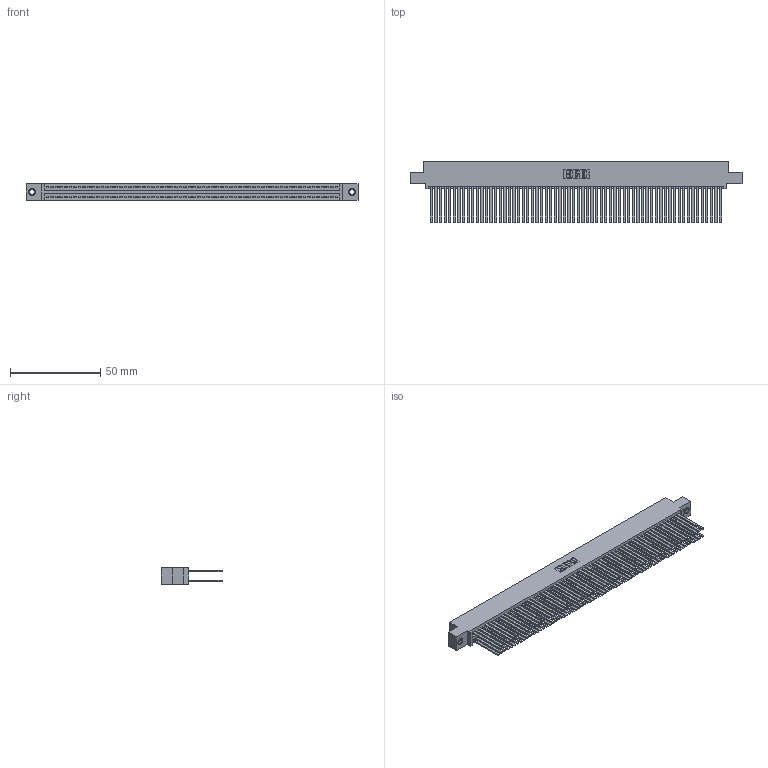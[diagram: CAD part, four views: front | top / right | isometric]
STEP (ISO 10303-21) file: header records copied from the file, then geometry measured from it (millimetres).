
FILE_DESCRIPTION (( 'STEP AP203' ), '1' );
FILE_NAME ('345-128-544-507.STEP', '2019-11-07T09:22:03', ( '' ), ( '' ), 'SwSTEP 2.0', 'SolidWorks 2016', '' );
FILE_SCHEMA (( 'CONFIG_CONTROL_DESIGN' ));
Length unit declared in the file: inch
Products named in the file (4): 345-128-544-507; 345-250-001_345-250-005-103; 345 Part_0.110 Offset - 0.156 Dia-TI; 345-292-001_345-293-144
Assembly tree (131 placements, depth 2):
  345-128-544-507
    345 Part_0.110 Offset - 0.156 Dia-TI
    345-292-001_345-293-144  x128
    345-250-001_345-250-005-103  x2
Bounding box: 183.77 x 33.96 x 9.4 mm (x, y, z)
Volume: 19763.2 mm3; surface area: 35019.1 mm2
Topology: 131 solids, 131 shells, 5822 faces, 17257 edges, 11326 vertices
Faces by surface type: plane 3828, cylinder 1978, cone 12, torus 4
Entity records: 48388 total; most frequent: CARTESIAN_POINT 8071, ORIENTED_EDGE 7998, DIRECTION 7113, EDGE_CURVE 3999, LINE 3595, VECTOR 3595, VERTEX_POINT 2660, AXIS2_PLACEMENT_3D 1759
